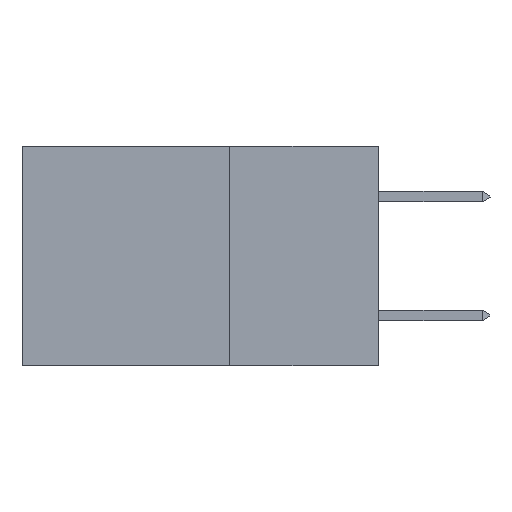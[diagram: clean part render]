
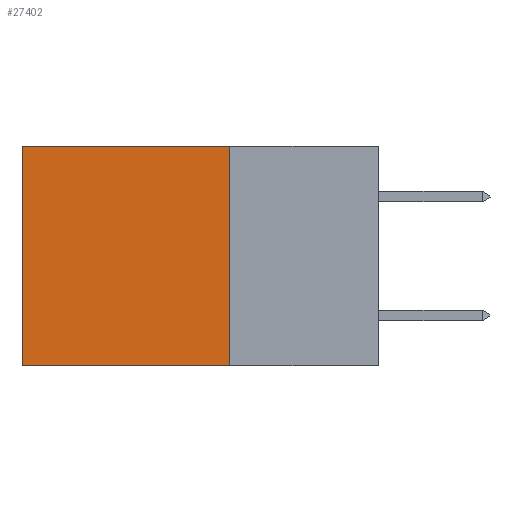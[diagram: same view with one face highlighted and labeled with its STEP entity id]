
A CAD part, left-side view. The second image highlights one B-rep face of the part: STEP entity #27402.
In plain terms, the highlighted planar face has unit normal (-1, 0, 0).
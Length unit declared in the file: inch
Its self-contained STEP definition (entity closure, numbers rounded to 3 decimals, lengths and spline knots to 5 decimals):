
#863 = LINE ( 'NONE', #8513, #8294 ) ;
#1142 = VERTEX_POINT ( 'NONE', #2846 ) ;
#2133 = LINE ( 'NONE', #23428, #26558 ) ;
#2846 = CARTESIAN_POINT ( 'NONE',  ( 0.298, 0.6, -0.37 ) ) ;
#3193 = LINE ( 'NONE', #23356, #7236 ) ;
#4300 = VERTEX_POINT ( 'NONE', #9019 ) ;
#6186 = DIRECTION ( 'NONE',  ( 0., 0., -1. ) ) ;
#6480 = VECTOR ( 'NONE', #12682, 39.37008 ) ;
#7236 = VECTOR ( 'NONE', #21113, 39.37008 ) ;
#7761 = EDGE_CURVE ( 'NONE', #20880, #15893, #2133, .T. ) ;
#7776 = CARTESIAN_POINT ( 'NONE',  ( 0.298, 0.25, 0. ) ) ;
#8294 = VECTOR ( 'NONE', #13472, 39.37008 ) ;
#8389 = EDGE_CURVE ( 'NONE', #15893, #1142, #12601, .T. ) ;
#8513 = CARTESIAN_POINT ( 'NONE',  ( 0.298, 0.6, 0. ) ) ;
#8632 = DIRECTION ( 'NONE',  ( 0., 0., -1. ) ) ;
#9019 = CARTESIAN_POINT ( 'NONE',  ( 0.298, 0.6, 0. ) ) ;
#11790 = EDGE_CURVE ( 'NONE', #4300, #1142, #863, .T. ) ;
#12601 = LINE ( 'NONE', #14768, #6480 ) ;
#12682 = DIRECTION ( 'NONE',  ( 0., 1., 0. ) ) ;
#13008 = DIRECTION ( 'NONE',  ( 1., 0., 0. ) ) ;
#13472 = DIRECTION ( 'NONE',  ( 0., 0., -1. ) ) ;
#14232 = AXIS2_PLACEMENT_3D ( 'NONE', #21625, #13008, #8632 ) ;
#14768 = CARTESIAN_POINT ( 'NONE',  ( 0.298, 0.25, -0.37 ) ) ;
#15893 = VERTEX_POINT ( 'NONE', #20622 ) ;
#16127 = EDGE_LOOP ( 'NONE', ( #21387, #17778, #16328, #17104 ) ) ;
#16328 = ORIENTED_EDGE ( 'NONE', *, *, #7761, .F. ) ;
#17104 = ORIENTED_EDGE ( 'NONE', *, *, #19153, .T. ) ;
#17299 = PLANE ( 'NONE',  #14232 ) ;
#17778 = ORIENTED_EDGE ( 'NONE', *, *, #8389, .F. ) ;
#19153 = EDGE_CURVE ( 'NONE', #20880, #4300, #3193, .T. ) ;
#20622 = CARTESIAN_POINT ( 'NONE',  ( 0.298, 0.25, -0.37 ) ) ;
#20880 = VERTEX_POINT ( 'NONE', #7776 ) ;
#21113 = DIRECTION ( 'NONE',  ( 0., 1., 0. ) ) ;
#21387 = ORIENTED_EDGE ( 'NONE', *, *, #11790, .T. ) ;
#21625 = CARTESIAN_POINT ( 'NONE',  ( 0.298, 0.25, 0. ) ) ;
#23356 = CARTESIAN_POINT ( 'NONE',  ( 0.298, 0.25, 0. ) ) ;
#23428 = CARTESIAN_POINT ( 'NONE',  ( 0.298, 0.25, 0. ) ) ;
#25534 = FACE_OUTER_BOUND ( 'NONE', #16127, .T. ) ;
#26558 = VECTOR ( 'NONE', #6186, 39.37008 ) ;
#27402 = ADVANCED_FACE ( 'NONE', ( #25534 ), #17299, .F. ) ;
